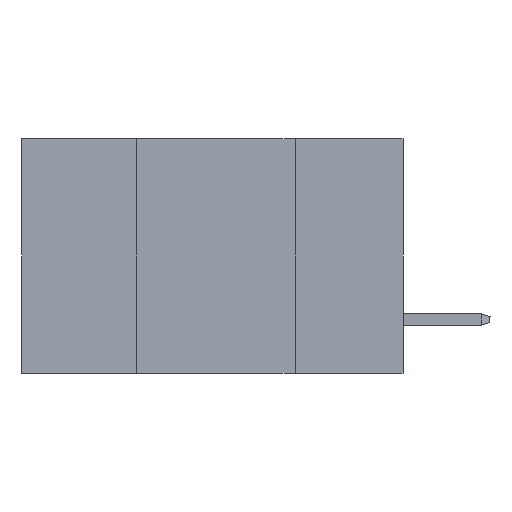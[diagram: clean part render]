
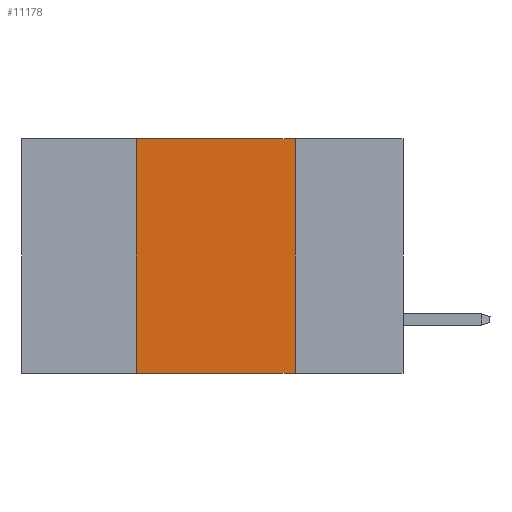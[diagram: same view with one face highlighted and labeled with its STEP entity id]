
A CAD part, left-side view. The second image highlights one B-rep face of the part: STEP entity #11178.
In plain terms, the highlighted planar face has unit normal (-1, 0, 0).
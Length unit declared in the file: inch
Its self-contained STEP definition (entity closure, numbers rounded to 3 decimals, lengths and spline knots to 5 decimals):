
#254 = CARTESIAN_POINT ( 'NONE',  ( 0., 0.42, 0. ) ) ;
#403 = ORIENTED_EDGE ( 'NONE', *, *, #4531, .F. ) ;
#844 = PLANE ( 'NONE',  #9803 ) ;
#1011 = VECTOR ( 'NONE', #6560, 39.37008 ) ;
#1098 = DIRECTION ( 'NONE',  ( 0., 0., -1. ) ) ;
#1332 = LINE ( 'NONE', #4412, #1011 ) ;
#1475 = ORIENTED_EDGE ( 'NONE', *, *, #2612, .T. ) ;
#1726 = VECTOR ( 'NONE', #6713, 39.37008 ) ;
#2139 = DIRECTION ( 'NONE',  ( 0., 0., 1. ) ) ;
#2582 = CARTESIAN_POINT ( 'NONE',  ( 0., 0.6, 0. ) ) ;
#2612 = EDGE_CURVE ( 'NONE', #13215, #6336, #1332, .T. ) ;
#3374 = VECTOR ( 'NONE', #1098, 39.37008 ) ;
#3697 = VECTOR ( 'NONE', #2139, 39.37008 ) ;
#4016 = FACE_OUTER_BOUND ( 'NONE', #8073, .T. ) ;
#4412 = CARTESIAN_POINT ( 'NONE',  ( 0., 0.6, -0.37 ) ) ;
#4531 = EDGE_CURVE ( 'NONE', #10956, #10176, #7726, .T. ) ;
#4944 = DIRECTION ( 'NONE',  ( 1., 0., 0. ) ) ;
#5262 = LINE ( 'NONE', #9503, #3697 ) ;
#5868 = CARTESIAN_POINT ( 'NONE',  ( 0., 0.6, 0. ) ) ;
#6122 = LINE ( 'NONE', #7097, #3374 ) ;
#6336 = VERTEX_POINT ( 'NONE', #13271 ) ;
#6508 = EDGE_CURVE ( 'NONE', #13215, #10956, #5262, .T. ) ;
#6560 = DIRECTION ( 'NONE',  ( 0., -1., 0. ) ) ;
#6713 = DIRECTION ( 'NONE',  ( 0., -1., 0. ) ) ;
#7057 = ORIENTED_EDGE ( 'NONE', *, *, #6508, .F. ) ;
#7097 = CARTESIAN_POINT ( 'NONE',  ( 0., 0.17, 0. ) ) ;
#7726 = LINE ( 'NONE', #2582, #1726 ) ;
#8073 = EDGE_LOOP ( 'NONE', ( #11584, #403, #7057, #1475 ) ) ;
#8258 = EDGE_CURVE ( 'NONE', #10176, #6336, #6122, .T. ) ;
#8659 = CARTESIAN_POINT ( 'NONE',  ( 0., 0.17, 0. ) ) ;
#9042 = DIRECTION ( 'NONE',  ( 0., 0., -1. ) ) ;
#9503 = CARTESIAN_POINT ( 'NONE',  ( 0., 0.42, 0. ) ) ;
#9803 = AXIS2_PLACEMENT_3D ( 'NONE', #5868, #4944, #9042 ) ;
#10176 = VERTEX_POINT ( 'NONE', #8659 ) ;
#10956 = VERTEX_POINT ( 'NONE', #254 ) ;
#11178 = ADVANCED_FACE ( 'NONE', ( #4016 ), #844, .F. ) ;
#11379 = CARTESIAN_POINT ( 'NONE',  ( 0., 0.42, -0.37 ) ) ;
#11584 = ORIENTED_EDGE ( 'NONE', *, *, #8258, .F. ) ;
#13215 = VERTEX_POINT ( 'NONE', #11379 ) ;
#13271 = CARTESIAN_POINT ( 'NONE',  ( 0., 0.17, -0.37 ) ) ;
